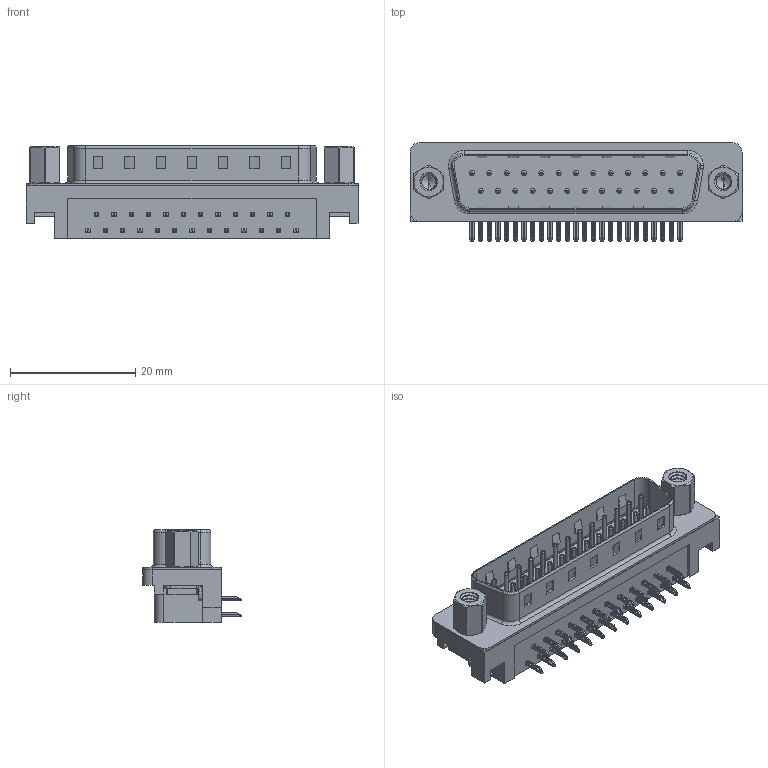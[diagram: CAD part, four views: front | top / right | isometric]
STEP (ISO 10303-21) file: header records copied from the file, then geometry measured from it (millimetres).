
FILE_DESCRIPTION (( 'STEP AP203' ), '1' );
FILE_NAME ('623-025-261-003.STEP', '2018-11-06T12:42:36', ( '' ), ( '' ), 'SwSTEP 2.0', 'SolidWorks 2016', '' );
FILE_SCHEMA (( 'CONFIG_CONTROL_DESIGN' ));
Length unit declared in the file: millimetre
Products named in the file (8): 623 4-40 Threaded Rivet; 623 4-40 Hex Standoff 5; 623-025-261-003; 623 Housing_25 Socket; 623 Shell_25 Socket; 623 Contact Bottom; 623 Contact Top; 623 Non Board Mount
Assembly tree (33 placements, depth 2):
  623-025-261-003
    623 Housing_25 Socket
    623 Shell_25 Socket
    623 Contact Bottom  x12
    623 Contact Top  x13
    623 Non Board Mount  x2
    623 4-40 Threaded Rivet  x2
    623 4-40 Hex Standoff 5  x2
Bounding box: 53.04 x 15.73 x 14.8 mm (x, y, z)
Volume: 4933.3 mm3; surface area: 7187.2 mm2
Topology: 33 solids, 33 shells, 2377 faces, 5907 edges, 3657 vertices
Faces by surface type: plane 1427, cylinder 717, torus 181, cone 34, bspline 18
Entity records: 26894 total; most frequent: CARTESIAN_POINT 8266, DIRECTION 3550, ORIENTED_EDGE 3528, EDGE_CURVE 1764, AXIS2_PLACEMENT_3D 1185, LINE 1180, VECTOR 1180, VERTEX_POINT 1133
